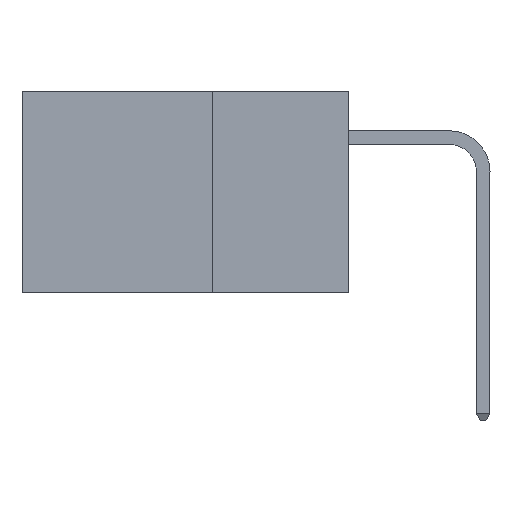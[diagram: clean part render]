
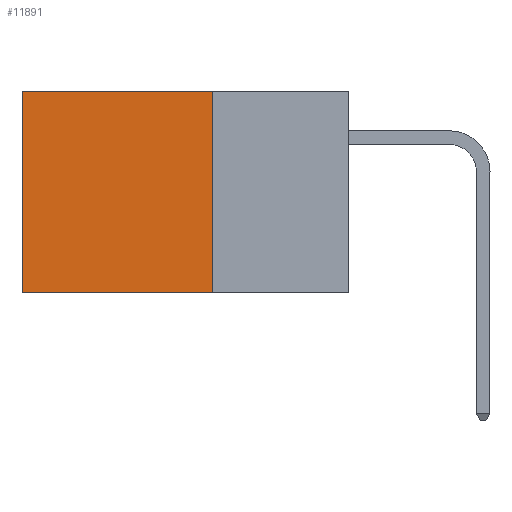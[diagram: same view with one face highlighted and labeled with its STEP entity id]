
A CAD part, left-side view. The second image highlights one B-rep face of the part: STEP entity #11891.
In plain terms, the highlighted planar face has unit normal (-1, 0, 0).
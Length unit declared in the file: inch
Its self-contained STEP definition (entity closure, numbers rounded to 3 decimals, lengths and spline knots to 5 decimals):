
#483 = DIRECTION ( 'NONE',  ( 0., 0., -1. ) ) ;
#817 = LINE ( 'NONE', #5711, #1345 ) ;
#1099 = ORIENTED_EDGE ( 'NONE', *, *, #2599, .T. ) ;
#1345 = VECTOR ( 'NONE', #11538, 39.37008 ) ;
#2134 = DIRECTION ( 'NONE',  ( 0., 1., 0. ) ) ;
#2234 = CARTESIAN_POINT ( 'NONE',  ( 0.2875, 0.25, 0. ) ) ;
#2264 = CARTESIAN_POINT ( 'NONE',  ( 0.2875, 0.25, 0. ) ) ;
#2452 = PLANE ( 'NONE',  #14078 ) ;
#2550 = EDGE_CURVE ( 'NONE', #6226, #11011, #817, .T. ) ;
#2599 = EDGE_CURVE ( 'NONE', #6226, #6704, #13329, .T. ) ;
#3522 = DIRECTION ( 'NONE',  ( 1., 0., 0. ) ) ;
#3782 = LINE ( 'NONE', #12462, #12648 ) ;
#4670 = VECTOR ( 'NONE', #13718, 39.37008 ) ;
#5288 = ORIENTED_EDGE ( 'NONE', *, *, #6002, .T. ) ;
#5711 = CARTESIAN_POINT ( 'NONE',  ( 0.2875, 0.25, 0. ) ) ;
#6002 = EDGE_CURVE ( 'NONE', #6704, #6646, #12146, .T. ) ;
#6226 = VERTEX_POINT ( 'NONE', #7078 ) ;
#6473 = CARTESIAN_POINT ( 'NONE',  ( 0.2875, 0.6, 0. ) ) ;
#6646 = VERTEX_POINT ( 'NONE', #9595 ) ;
#6704 = VERTEX_POINT ( 'NONE', #6473 ) ;
#7078 = CARTESIAN_POINT ( 'NONE',  ( 0.2875, 0.25, 0. ) ) ;
#8355 = VECTOR ( 'NONE', #483, 39.37008 ) ;
#9595 = CARTESIAN_POINT ( 'NONE',  ( 0.2875, 0.6, -0.37 ) ) ;
#10602 = CARTESIAN_POINT ( 'NONE',  ( 0.2875, 0.6, 0. ) ) ;
#10703 = EDGE_LOOP ( 'NONE', ( #5288, #13732, #14362, #1099 ) ) ;
#11011 = VERTEX_POINT ( 'NONE', #13714 ) ;
#11538 = DIRECTION ( 'NONE',  ( 0., 0., -1. ) ) ;
#11891 = ADVANCED_FACE ( 'NONE', ( #13655 ), #2452, .F. ) ;
#12146 = LINE ( 'NONE', #10602, #8355 ) ;
#12462 = CARTESIAN_POINT ( 'NONE',  ( 0.2875, 0.25, -0.37 ) ) ;
#12648 = VECTOR ( 'NONE', #2134, 39.37008 ) ;
#12744 = EDGE_CURVE ( 'NONE', #11011, #6646, #3782, .T. ) ;
#13329 = LINE ( 'NONE', #2264, #4670 ) ;
#13655 = FACE_OUTER_BOUND ( 'NONE', #10703, .T. ) ;
#13714 = CARTESIAN_POINT ( 'NONE',  ( 0.2875, 0.25, -0.37 ) ) ;
#13718 = DIRECTION ( 'NONE',  ( 0., 1., 0. ) ) ;
#13732 = ORIENTED_EDGE ( 'NONE', *, *, #12744, .F. ) ;
#14078 = AXIS2_PLACEMENT_3D ( 'NONE', #2234, #3522, #15007 ) ;
#14362 = ORIENTED_EDGE ( 'NONE', *, *, #2550, .F. ) ;
#15007 = DIRECTION ( 'NONE',  ( 0., 0., -1. ) ) ;
